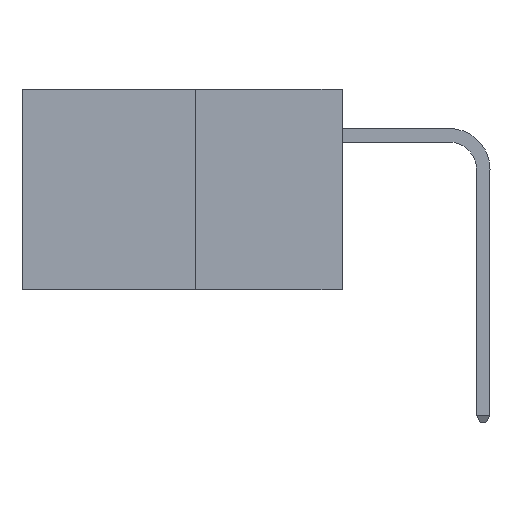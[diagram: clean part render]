
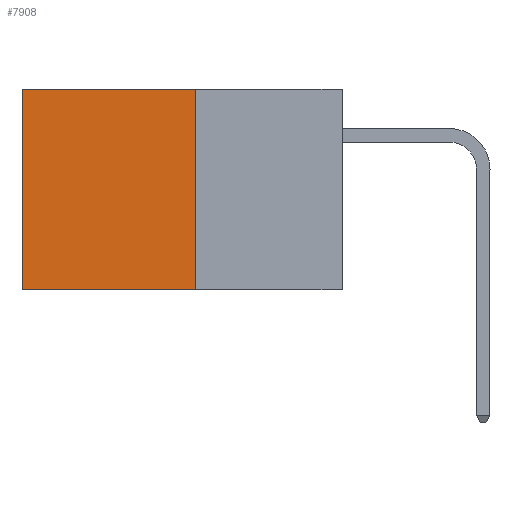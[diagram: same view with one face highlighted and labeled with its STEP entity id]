
A CAD part, left-side view. The second image highlights one B-rep face of the part: STEP entity #7908.
In plain terms, the highlighted planar face has unit normal (-1, 0, 0).
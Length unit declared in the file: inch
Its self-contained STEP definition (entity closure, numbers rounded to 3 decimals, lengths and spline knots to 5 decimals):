
#749 = EDGE_CURVE ( 'NONE', #4374, #18115, #11225, .T. ) ;
#755 = LINE ( 'NONE', #21514, #5438 ) ;
#1155 = ORIENTED_EDGE ( 'NONE', *, *, #21373, .T. ) ;
#1583 = VERTEX_POINT ( 'NONE', #12399 ) ;
#4374 = VERTEX_POINT ( 'NONE', #5989 ) ;
#5438 = VECTOR ( 'NONE', #23393, 39.37008 ) ;
#5989 = CARTESIAN_POINT ( 'NONE',  ( 0.277, 0.27, 0. ) ) ;
#6192 = EDGE_CURVE ( 'NONE', #15074, #1583, #755, .T. ) ;
#7172 = PLANE ( 'NONE',  #22960 ) ;
#7908 = ADVANCED_FACE ( 'NONE', ( #16775 ), #7172, .F. ) ;
#8069 = DIRECTION ( 'NONE',  ( 0., 0., -1. ) ) ;
#9159 = CARTESIAN_POINT ( 'NONE',  ( 0.277, 0.27, -0.37 ) ) ;
#11109 = DIRECTION ( 'NONE',  ( 1., 0., 0. ) ) ;
#11225 = LINE ( 'NONE', #24952, #16512 ) ;
#11737 = VECTOR ( 'NONE', #16526, 39.37008 ) ;
#11832 = EDGE_CURVE ( 'NONE', #4374, #15074, #22548, .T. ) ;
#12347 = CARTESIAN_POINT ( 'NONE',  ( 0.277, 0.27, -0.37 ) ) ;
#12399 = CARTESIAN_POINT ( 'NONE',  ( 0.277, 0.59, -0.37 ) ) ;
#12537 = CARTESIAN_POINT ( 'NONE',  ( 0.277, 0.27, -0.37 ) ) ;
#13954 = ORIENTED_EDGE ( 'NONE', *, *, #749, .T. ) ;
#15074 = VERTEX_POINT ( 'NONE', #12347 ) ;
#15922 = CARTESIAN_POINT ( 'NONE',  ( 0.277, 0.59, -0.37 ) ) ;
#16085 = DIRECTION ( 'NONE',  ( 0., 1., 0. ) ) ;
#16396 = ORIENTED_EDGE ( 'NONE', *, *, #6192, .F. ) ;
#16512 = VECTOR ( 'NONE', #16085, 39.37008 ) ;
#16526 = DIRECTION ( 'NONE',  ( 0., 0., -1. ) ) ;
#16775 = FACE_OUTER_BOUND ( 'NONE', #19819, .T. ) ;
#17309 = CARTESIAN_POINT ( 'NONE',  ( 0.277, 0.59, 0. ) ) ;
#17838 = VECTOR ( 'NONE', #8069, 39.37008 ) ;
#18115 = VERTEX_POINT ( 'NONE', #17309 ) ;
#18453 = LINE ( 'NONE', #15922, #17838 ) ;
#18515 = ORIENTED_EDGE ( 'NONE', *, *, #11832, .F. ) ;
#19819 = EDGE_LOOP ( 'NONE', ( #1155, #16396, #18515, #13954 ) ) ;
#21373 = EDGE_CURVE ( 'NONE', #18115, #1583, #18453, .T. ) ;
#21514 = CARTESIAN_POINT ( 'NONE',  ( 0.277, 0.27, -0.37 ) ) ;
#22548 = LINE ( 'NONE', #12537, #11737 ) ;
#22960 = AXIS2_PLACEMENT_3D ( 'NONE', #9159, #11109, #24514 ) ;
#23393 = DIRECTION ( 'NONE',  ( 0., 1., 0. ) ) ;
#24514 = DIRECTION ( 'NONE',  ( 0., 0., -1. ) ) ;
#24952 = CARTESIAN_POINT ( 'NONE',  ( 0.277, 0.27, 0. ) ) ;
